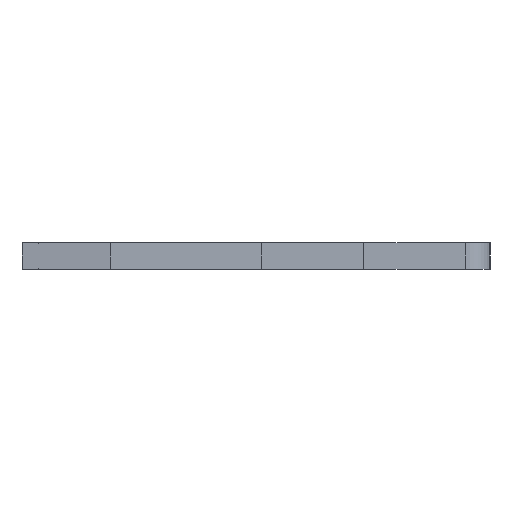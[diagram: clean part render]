
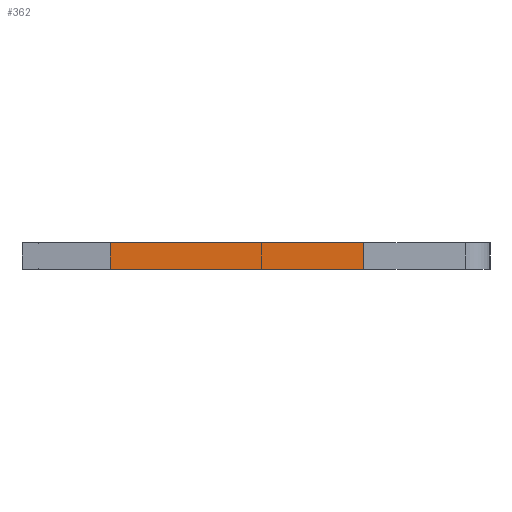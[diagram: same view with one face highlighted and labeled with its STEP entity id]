
A CAD part, left-side view. The second image highlights one B-rep face of the part: STEP entity #362.
In plain terms, the highlighted face is planar.
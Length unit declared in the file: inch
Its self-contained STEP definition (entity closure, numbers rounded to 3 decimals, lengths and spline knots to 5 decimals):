
#22 = LINE ( 'NONE', #2410, #2326 ) ;
#64 = DIRECTION ( 'NONE',  ( 0., 1., 0. ) ) ;
#157 = DIRECTION ( 'NONE',  ( 0., 0., 1. ) ) ;
#242 = VECTOR ( 'NONE', #963, 39.37008 ) ;
#286 = CARTESIAN_POINT ( 'NONE',  ( 0.013, 0.146, -0.0575 ) ) ;
#336 = CARTESIAN_POINT ( 'NONE',  ( 0.013, 0.146, -0.0575 ) ) ;
#362 = ADVANCED_FACE ( 'NONE', ( #2508 ), #954, .F. ) ;
#386 = EDGE_CURVE ( 'NONE', #1963, #1935, #2293, .T. ) ;
#435 = CARTESIAN_POINT ( 'NONE',  ( 0.013, 0.146, -0.0575 ) ) ;
#450 = ORIENTED_EDGE ( 'NONE', *, *, #1287, .F. ) ;
#467 = LINE ( 'NONE', #2163, #242 ) ;
#503 = AXIS2_PLACEMENT_3D ( 'NONE', #336, #157, #1701 ) ;
#583 = EDGE_CURVE ( 'NONE', #1935, #793, #467, .T. ) ;
#595 = VERTEX_POINT ( 'NONE', #435 ) ;
#728 = VECTOR ( 'NONE', #921, 39.37008 ) ;
#735 = ORIENTED_EDGE ( 'NONE', *, *, #386, .T. ) ;
#793 = VERTEX_POINT ( 'NONE', #1356 ) ;
#921 = DIRECTION ( 'NONE',  ( -1., 0., 0. ) ) ;
#954 = PLANE ( 'NONE',  #503 ) ;
#963 = DIRECTION ( 'NONE',  ( 0., 1., 0. ) ) ;
#1003 = EDGE_CURVE ( 'NONE', #1963, #595, #22, .T. ) ;
#1072 = DIRECTION ( 'NONE',  ( -1., 0., 0. ) ) ;
#1115 = CARTESIAN_POINT ( 'NONE',  ( 0.013, -0.099, -0.0575 ) ) ;
#1287 = EDGE_CURVE ( 'NONE', #595, #793, #1504, .T. ) ;
#1356 = CARTESIAN_POINT ( 'NONE',  ( -0.013, 0.146, -0.0575 ) ) ;
#1482 = ORIENTED_EDGE ( 'NONE', *, *, #1003, .F. ) ;
#1504 = LINE ( 'NONE', #286, #2393 ) ;
#1511 = ORIENTED_EDGE ( 'NONE', *, *, #583, .T. ) ;
#1672 = CARTESIAN_POINT ( 'NONE',  ( 0.013, -0.099, -0.0575 ) ) ;
#1701 = DIRECTION ( 'NONE',  ( 1., 0., 0. ) ) ;
#1935 = VERTEX_POINT ( 'NONE', #2287 ) ;
#1963 = VERTEX_POINT ( 'NONE', #1672 ) ;
#2163 = CARTESIAN_POINT ( 'NONE',  ( -0.013, 0.146, -0.0575 ) ) ;
#2187 = EDGE_LOOP ( 'NONE', ( #1511, #450, #1482, #735 ) ) ;
#2287 = CARTESIAN_POINT ( 'NONE',  ( -0.013, -0.099, -0.0575 ) ) ;
#2293 = LINE ( 'NONE', #1115, #728 ) ;
#2326 = VECTOR ( 'NONE', #64, 39.37008 ) ;
#2393 = VECTOR ( 'NONE', #1072, 39.37008 ) ;
#2410 = CARTESIAN_POINT ( 'NONE',  ( 0.013, 0.146, -0.0575 ) ) ;
#2508 = FACE_OUTER_BOUND ( 'NONE', #2187, .T. ) ;
